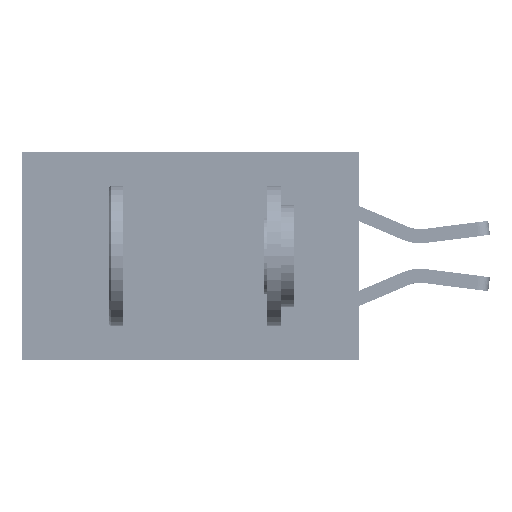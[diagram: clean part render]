
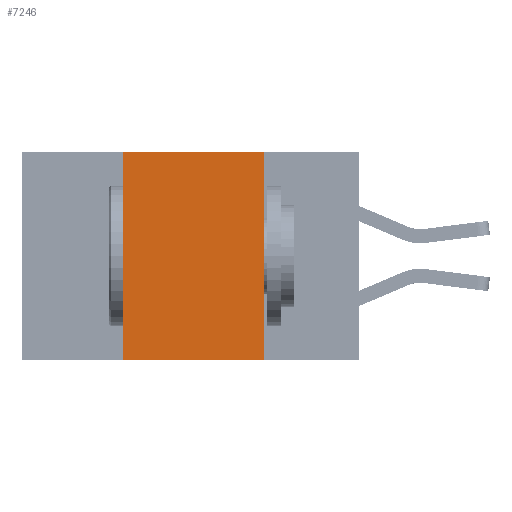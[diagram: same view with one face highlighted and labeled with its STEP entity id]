
A CAD part, left-side view. The second image highlights one B-rep face of the part: STEP entity #7246.
In plain terms, the highlighted planar face has unit normal (-1, 0, 0).
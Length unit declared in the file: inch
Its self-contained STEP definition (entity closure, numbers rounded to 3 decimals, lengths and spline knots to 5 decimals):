
#463 = CARTESIAN_POINT ( 'NONE',  ( 0., 0.6, 0. ) ) ;
#933 = ORIENTED_EDGE ( 'NONE', *, *, #24865, .F. ) ;
#2717 = CARTESIAN_POINT ( 'NONE',  ( 0., 0.17, 0. ) ) ;
#3096 = VERTEX_POINT ( 'NONE', #24845 ) ;
#5611 = CARTESIAN_POINT ( 'NONE',  ( 0., 0.17, -0.37 ) ) ;
#6463 = DIRECTION ( 'NONE',  ( 0., 0., -1. ) ) ;
#6674 = VECTOR ( 'NONE', #13811, 39.37008 ) ;
#7246 = ADVANCED_FACE ( 'NONE', ( #11594 ), #29599, .F. ) ;
#9713 = CARTESIAN_POINT ( 'NONE',  ( 0., 0.6, 0. ) ) ;
#10110 = CARTESIAN_POINT ( 'NONE',  ( 0., 0.6, -0.37 ) ) ;
#11132 = EDGE_LOOP ( 'NONE', ( #46341, #933, #30886, #14561 ) ) ;
#11594 = FACE_OUTER_BOUND ( 'NONE', #11132, .T. ) ;
#13811 = DIRECTION ( 'NONE',  ( 0., -1., 0. ) ) ;
#14561 = ORIENTED_EDGE ( 'NONE', *, *, #35766, .T. ) ;
#15297 = VECTOR ( 'NONE', #43797, 39.37008 ) ;
#18809 = LINE ( 'NONE', #9713, #45857 ) ;
#20796 = VERTEX_POINT ( 'NONE', #5611 ) ;
#23091 = LINE ( 'NONE', #2717, #40747 ) ;
#24845 = CARTESIAN_POINT ( 'NONE',  ( 0., 0.42, 0. ) ) ;
#24865 = EDGE_CURVE ( 'NONE', #3096, #29175, #18809, .T. ) ;
#26916 = EDGE_CURVE ( 'NONE', #31214, #3096, #34282, .T. ) ;
#29175 = VERTEX_POINT ( 'NONE', #37834 ) ;
#29599 = PLANE ( 'NONE',  #38616 ) ;
#30886 = ORIENTED_EDGE ( 'NONE', *, *, #26916, .F. ) ;
#31214 = VERTEX_POINT ( 'NONE', #44972 ) ;
#33115 = EDGE_CURVE ( 'NONE', #29175, #20796, #23091, .T. ) ;
#33127 = DIRECTION ( 'NONE',  ( 0., 0., -1. ) ) ;
#34282 = LINE ( 'NONE', #40297, #15297 ) ;
#34848 = DIRECTION ( 'NONE',  ( 0., -1., 0. ) ) ;
#35413 = LINE ( 'NONE', #10110, #6674 ) ;
#35766 = EDGE_CURVE ( 'NONE', #31214, #20796, #35413, .T. ) ;
#37834 = CARTESIAN_POINT ( 'NONE',  ( 0., 0.17, 0. ) ) ;
#38616 = AXIS2_PLACEMENT_3D ( 'NONE', #463, #40018, #33127 ) ;
#40018 = DIRECTION ( 'NONE',  ( 1., 0., 0. ) ) ;
#40297 = CARTESIAN_POINT ( 'NONE',  ( 0., 0.42, 0. ) ) ;
#40747 = VECTOR ( 'NONE', #6463, 39.37008 ) ;
#43797 = DIRECTION ( 'NONE',  ( 0., 0., 1. ) ) ;
#44972 = CARTESIAN_POINT ( 'NONE',  ( 0., 0.42, -0.37 ) ) ;
#45857 = VECTOR ( 'NONE', #34848, 39.37008 ) ;
#46341 = ORIENTED_EDGE ( 'NONE', *, *, #33115, .F. ) ;
